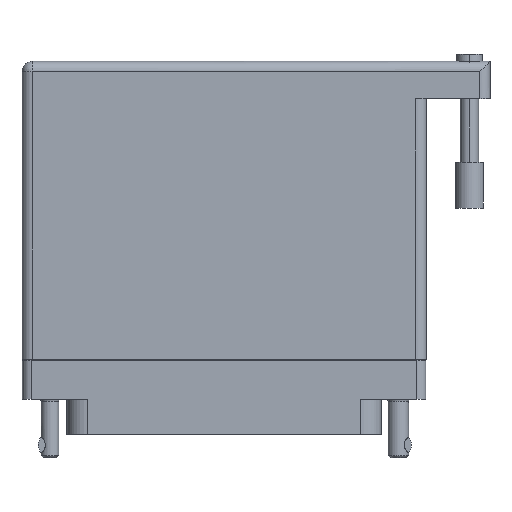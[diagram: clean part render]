
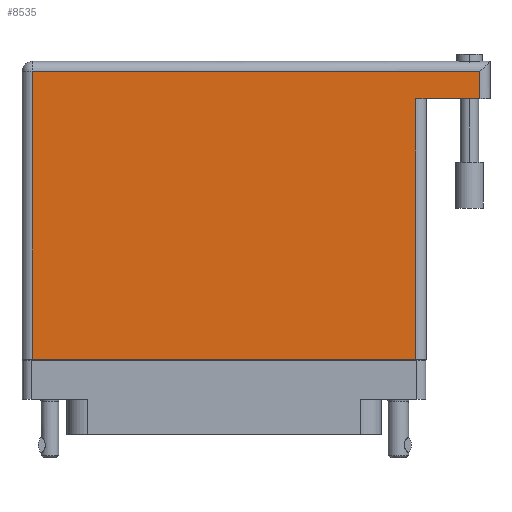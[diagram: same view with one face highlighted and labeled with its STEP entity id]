
A CAD part, front view. The second image highlights one B-rep face of the part: STEP entity #8535.
In plain terms, the highlighted face is planar.
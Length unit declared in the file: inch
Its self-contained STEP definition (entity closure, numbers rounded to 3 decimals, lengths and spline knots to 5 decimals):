
#3955 = CARTESIAN_POINT ( 'NONE',  ( -1.3775, 1.93, 0.765 ) ) ;
#8535 = ADVANCED_FACE ( 'NONE', ( #46991 ), #93289, .F. ) ;
#8804 = VECTOR ( 'NONE', #32236, 39.37008 ) ;
#9943 = CARTESIAN_POINT ( 'NONE',  ( 1.3075, -0.1, 0.765 ) ) ;
#12207 = ORIENTED_EDGE ( 'NONE', *, *, #13175, .F. ) ;
#12345 = VECTOR ( 'NONE', #49159, 39.37008 ) ;
#13175 = EDGE_CURVE ( 'NONE', #73868, #16552, #28596, .T. ) ;
#13671 = CARTESIAN_POINT ( 'NONE',  ( 1.7425, 1.674, 0.765 ) ) ;
#13751 = DIRECTION ( 'NONE',  ( 1., 0., 0. ) ) ;
#16552 = VERTEX_POINT ( 'NONE', #85230 ) ;
#18521 = DIRECTION ( 'NONE',  ( 0., 0., -1. ) ) ;
#19920 = ORIENTED_EDGE ( 'NONE', *, *, #82395, .T. ) ;
#20815 = VERTEX_POINT ( 'NONE', #9943 ) ;
#23628 = LINE ( 'NONE', #73965, #28325 ) ;
#24048 = VECTOR ( 'NONE', #73224, 39.37008 ) ;
#28325 = VECTOR ( 'NONE', #13751, 39.37008 ) ;
#28335 = CARTESIAN_POINT ( 'NONE',  ( 1.7425, 1.86, 0.765 ) ) ;
#28596 = LINE ( 'NONE', #48428, #8804 ) ;
#31702 = EDGE_LOOP ( 'NONE', ( #81249, #83187, #12207, #19920, #71739, #46696 ) ) ;
#32172 = DIRECTION ( 'NONE',  ( 0., -1., 0. ) ) ;
#32236 = DIRECTION ( 'NONE',  ( -1., 0., 0. ) ) ;
#32485 = CARTESIAN_POINT ( 'NONE',  ( -1.3075, -0.1, 0.765 ) ) ;
#39096 = CARTESIAN_POINT ( 'NONE',  ( 1.7425, 1.93, 0.765 ) ) ;
#39176 = LINE ( 'NONE', #39096, #12345 ) ;
#43890 = EDGE_CURVE ( 'NONE', #51243, #54214, #79178, .T. ) ;
#45608 = CARTESIAN_POINT ( 'NONE',  ( -1.3075, 1.86, 0.765 ) ) ;
#46696 = ORIENTED_EDGE ( 'NONE', *, *, #43890, .T. ) ;
#46991 = FACE_OUTER_BOUND ( 'NONE', #31702, .T. ) ;
#48428 = CARTESIAN_POINT ( 'NONE',  ( 1.8125, 1.674, 0.765 ) ) ;
#49159 = DIRECTION ( 'NONE',  ( 0., 1., 0. ) ) ;
#50843 = CARTESIAN_POINT ( 'NONE',  ( 1.3075, 1.674, 0.765 ) ) ;
#50935 = LINE ( 'NONE', #58913, #24048 ) ;
#51243 = VERTEX_POINT ( 'NONE', #45608 ) ;
#51712 = EDGE_CURVE ( 'NONE', #92360, #51243, #50935, .T. ) ;
#54214 = VERTEX_POINT ( 'NONE', #72431 ) ;
#56053 = DIRECTION ( 'NONE',  ( -1., 0., 0. ) ) ;
#58913 = CARTESIAN_POINT ( 'NONE',  ( -1.3775, 1.86, 0.765 ) ) ;
#59379 = VECTOR ( 'NONE', #80042, 39.37008 ) ;
#65159 = AXIS2_PLACEMENT_3D ( 'NONE', #3955, #18521, #56053 ) ;
#71739 = ORIENTED_EDGE ( 'NONE', *, *, #51712, .T. ) ;
#72431 = CARTESIAN_POINT ( 'NONE',  ( -1.3075, -0.1, 0.765 ) ) ;
#73224 = DIRECTION ( 'NONE',  ( -1., 0., 0. ) ) ;
#73868 = VERTEX_POINT ( 'NONE', #13671 ) ;
#73965 = CARTESIAN_POINT ( 'NONE',  ( -1.3775, -0.1, 0.765 ) ) ;
#75153 = EDGE_CURVE ( 'NONE', #54214, #20815, #23628, .T. ) ;
#79054 = EDGE_CURVE ( 'NONE', #20815, #16552, #84904, .T. ) ;
#79178 = LINE ( 'NONE', #32485, #95430 ) ;
#80042 = DIRECTION ( 'NONE',  ( 0., 1., 0. ) ) ;
#81249 = ORIENTED_EDGE ( 'NONE', *, *, #75153, .T. ) ;
#82395 = EDGE_CURVE ( 'NONE', #73868, #92360, #39176, .T. ) ;
#83187 = ORIENTED_EDGE ( 'NONE', *, *, #79054, .T. ) ;
#84904 = LINE ( 'NONE', #50843, #59379 ) ;
#85230 = CARTESIAN_POINT ( 'NONE',  ( 1.3075, 1.674, 0.765 ) ) ;
#92360 = VERTEX_POINT ( 'NONE', #28335 ) ;
#93289 = PLANE ( 'NONE',  #65159 ) ;
#95430 = VECTOR ( 'NONE', #32172, 39.37008 ) ;
